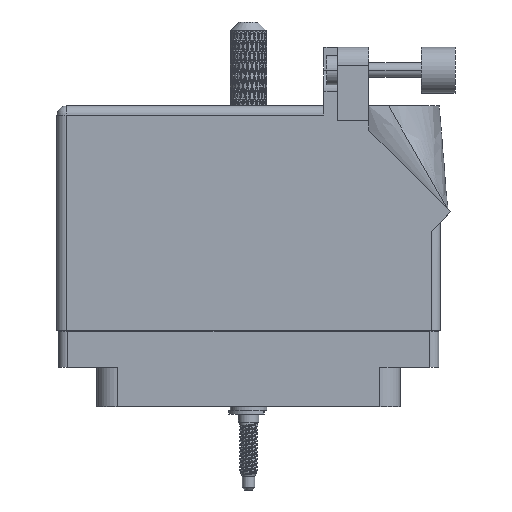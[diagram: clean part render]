
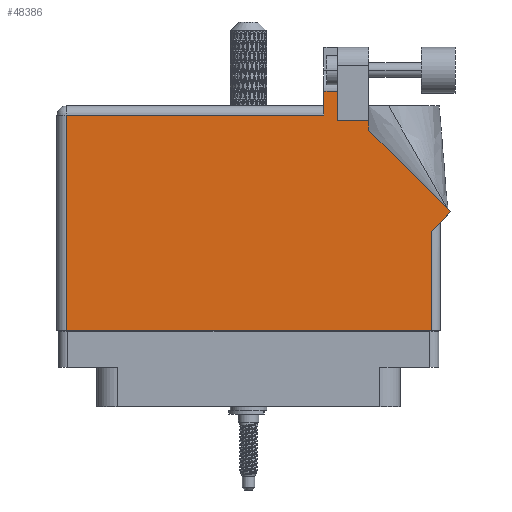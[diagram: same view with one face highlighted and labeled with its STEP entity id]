
A CAD part, front view. The second image highlights one B-rep face of the part: STEP entity #48386.
In plain terms, the highlighted face is planar.
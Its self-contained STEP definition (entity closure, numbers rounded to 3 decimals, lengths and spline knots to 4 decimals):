
#59 = CARTESIAN_POINT ( 'NONE',  ( 0.607, 1.33, 0.455 ) ) ;
#232 = CARTESIAN_POINT ( 'NONE',  ( 0.82, 1.2644, 0.455 ) ) ;
#2390 = CARTESIAN_POINT ( 'NONE',  ( -1.306, 1.368, 0.455 ) ) ;
#3736 = EDGE_CURVE ( 'NONE', #61691, #109237, #47287, .T. ) ;
#3992 = ORIENTED_EDGE ( 'NONE', *, *, #78585, .T. ) ;
#4320 = CARTESIAN_POINT ( 'NONE',  ( 1.306, 0.637, 0.455 ) ) ;
#4698 = DIRECTION ( 'NONE',  ( 0.707, 0.707, 0. ) ) ;
#7822 = VECTOR ( 'NONE', #4698, 39.3701 ) ;
#9705 = CARTESIAN_POINT ( 'NONE',  ( -1.244, -0.1, 0.455 ) ) ;
#10394 = FACE_OUTER_BOUND ( 'NONE', #48895, .T. ) ;
#14518 = CARTESIAN_POINT ( 'NONE',  ( 0.607, 1.5315, 0.455 ) ) ;
#15095 = LINE ( 'NONE', #9705, #73523 ) ;
#18359 = CARTESIAN_POINT ( 'NONE',  ( 0.9378, 1.5315, 0.455 ) ) ;
#18712 = VECTOR ( 'NONE', #28057, 39.3701 ) ;
#20585 = LINE ( 'NONE', #67515, #47666 ) ;
#21360 = DIRECTION ( 'NONE',  ( 1., 0., 0. ) ) ;
#22514 = EDGE_CURVE ( 'NONE', #67063, #109339, #113398, .T. ) ;
#27080 = CARTESIAN_POINT ( 'NONE',  ( 0.607, 1.33, 0.455 ) ) ;
#28057 = DIRECTION ( 'NONE',  ( 0., 1., 0. ) ) ;
#30758 = CARTESIAN_POINT ( 'NONE',  ( 0.82, 1.2644, 0.455 ) ) ;
#30826 = VERTEX_POINT ( 'NONE', #104922 ) ;
#31681 = LINE ( 'NONE', #59, #98540 ) ;
#32064 = CARTESIAN_POINT ( 'NONE',  ( 0.82, 1.33, 0.455 ) ) ;
#32399 = ORIENTED_EDGE ( 'NONE', *, *, #3736, .T. ) ;
#33584 = LINE ( 'NONE', #4320, #7822 ) ;
#41419 = ORIENTED_EDGE ( 'NONE', *, *, #101642, .T. ) ;
#41823 = CARTESIAN_POINT ( 'NONE',  ( 1.244, 0.575, 0.455 ) ) ;
#42083 = ORIENTED_EDGE ( 'NONE', *, *, #82494, .T. ) ;
#42709 = CARTESIAN_POINT ( 'NONE',  ( 0.513, 1.5315, 0.455 ) ) ;
#42771 = PLANE ( 'NONE',  #97052 ) ;
#45861 = DIRECTION ( 'NONE',  ( 0., 1., 0. ) ) ;
#47209 = ORIENTED_EDGE ( 'NONE', *, *, #81550, .T. ) ;
#47287 = LINE ( 'NONE', #92530, #18712 ) ;
#47666 = VECTOR ( 'NONE', #21360, 39.3701 ) ;
#48386 = ADVANCED_FACE ( 'NONE', ( #10394 ), #42771, .F. ) ;
#48738 = ORIENTED_EDGE ( 'NONE', *, *, #22514, .T. ) ;
#48895 = EDGE_LOOP ( 'NONE', ( #85303, #66756, #41419, #48738, #47209, #42083, #32399, #117106, #99209, #3992, #75178 ) ) ;
#49077 = CARTESIAN_POINT ( 'NONE',  ( 1.3767, 0.7077, 0.455 ) ) ;
#50662 = CARTESIAN_POINT ( 'NONE',  ( -1.306, 1.43, 0.455 ) ) ;
#52546 = VECTOR ( 'NONE', #84088, 39.3701 ) ;
#52625 = EDGE_CURVE ( 'NONE', #106178, #61860, #98068, .T. ) ;
#52985 = DIRECTION ( 'NONE',  ( -1., 0., 0. ) ) ;
#54985 = CARTESIAN_POINT ( 'NONE',  ( 0.513, 1.368, 0.455 ) ) ;
#59073 = DIRECTION ( 'NONE',  ( -1., 0., 0. ) ) ;
#59782 = VERTEX_POINT ( 'NONE', #77136 ) ;
#61691 = VERTEX_POINT ( 'NONE', #84139 ) ;
#61860 = VERTEX_POINT ( 'NONE', #42709 ) ;
#63987 = DIRECTION ( 'NONE',  ( 0., -1., 0. ) ) ;
#64012 = VECTOR ( 'NONE', #59073, 39.3701 ) ;
#64426 = EDGE_CURVE ( 'NONE', #59782, #87835, #98193, .T. ) ;
#65354 = LINE ( 'NONE', #30758, #52546 ) ;
#66756 = ORIENTED_EDGE ( 'NONE', *, *, #52625, .T. ) ;
#67063 = VERTEX_POINT ( 'NONE', #54985 ) ;
#67429 = DIRECTION ( 'NONE',  ( -0.707, 0.707, 0. ) ) ;
#67515 = CARTESIAN_POINT ( 'NONE',  ( -1.306, -0.1, 0.455 ) ) ;
#67805 = VERTEX_POINT ( 'NONE', #72189 ) ;
#69648 = LINE ( 'NONE', #49077, #75397 ) ;
#70168 = DIRECTION ( 'NONE',  ( -1., 0., 0. ) ) ;
#70297 = VECTOR ( 'NONE', #63987, 39.3701 ) ;
#70821 = CARTESIAN_POINT ( 'NONE',  ( -1.244, 1.368, 0.455 ) ) ;
#72068 = EDGE_CURVE ( 'NONE', #87835, #106178, #31681, .T. ) ;
#72189 = CARTESIAN_POINT ( 'NONE',  ( 1.3767, 0.7077, 0.455 ) ) ;
#73523 = VECTOR ( 'NONE', #110900, 39.3701 ) ;
#75178 = ORIENTED_EDGE ( 'NONE', *, *, #64426, .T. ) ;
#75397 = VECTOR ( 'NONE', #67429, 39.3701 ) ;
#77136 = CARTESIAN_POINT ( 'NONE',  ( 0.82, 1.33, 0.455 ) ) ;
#78585 = EDGE_CURVE ( 'NONE', #112927, #59782, #65354, .T. ) ;
#81550 = EDGE_CURVE ( 'NONE', #109339, #30826, #15095, .T. ) ;
#82118 = EDGE_CURVE ( 'NONE', #109237, #67805, #33584, .T. ) ;
#82494 = EDGE_CURVE ( 'NONE', #30826, #61691, #20585, .T. ) ;
#84088 = DIRECTION ( 'NONE',  ( 0., 1., 0. ) ) ;
#84139 = CARTESIAN_POINT ( 'NONE',  ( 1.244, -0.1, 0.455 ) ) ;
#84448 = DIRECTION ( 'NONE',  ( -1., 0., 0. ) ) ;
#85303 = ORIENTED_EDGE ( 'NONE', *, *, #72068, .T. ) ;
#87835 = VERTEX_POINT ( 'NONE', #27080 ) ;
#88846 = LINE ( 'NONE', #99060, #70297 ) ;
#92530 = CARTESIAN_POINT ( 'NONE',  ( 1.244, 0.637, 0.455 ) ) ;
#97052 = AXIS2_PLACEMENT_3D ( 'NONE', #50662, #115567, #70168 ) ;
#98068 = LINE ( 'NONE', #18359, #112547 ) ;
#98193 = LINE ( 'NONE', #32064, #64012 ) ;
#98540 = VECTOR ( 'NONE', #45861, 39.3701 ) ;
#99060 = CARTESIAN_POINT ( 'NONE',  ( 0.513, 1.43, 0.455 ) ) ;
#99209 = ORIENTED_EDGE ( 'NONE', *, *, #106560, .T. ) ;
#101642 = EDGE_CURVE ( 'NONE', #61860, #67063, #88846, .T. ) ;
#103442 = VECTOR ( 'NONE', #84448, 39.3701 ) ;
#104922 = CARTESIAN_POINT ( 'NONE',  ( -1.244, -0.1, 0.455 ) ) ;
#106178 = VERTEX_POINT ( 'NONE', #14518 ) ;
#106560 = EDGE_CURVE ( 'NONE', #67805, #112927, #69648, .T. ) ;
#109237 = VERTEX_POINT ( 'NONE', #41823 ) ;
#109339 = VERTEX_POINT ( 'NONE', #70821 ) ;
#110900 = DIRECTION ( 'NONE',  ( 0., -1., 0. ) ) ;
#112547 = VECTOR ( 'NONE', #52985, 39.3701 ) ;
#112927 = VERTEX_POINT ( 'NONE', #232 ) ;
#113398 = LINE ( 'NONE', #2390, #103442 ) ;
#115567 = DIRECTION ( 'NONE',  ( 0., 0., -1. ) ) ;
#117106 = ORIENTED_EDGE ( 'NONE', *, *, #82118, .T. ) ;
